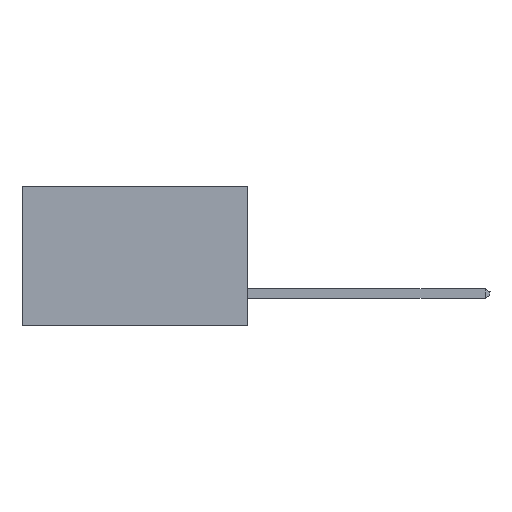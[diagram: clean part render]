
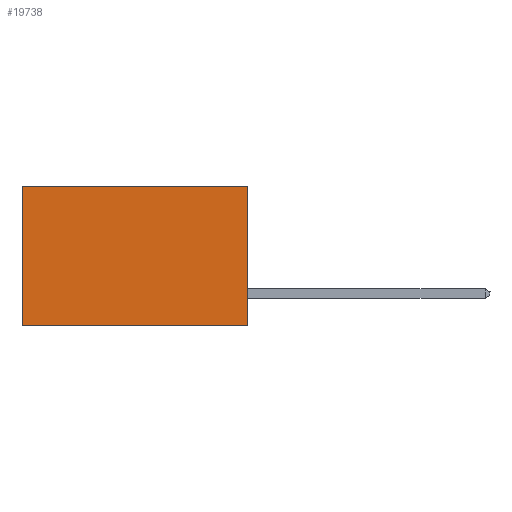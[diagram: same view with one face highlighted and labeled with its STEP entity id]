
A CAD part, left-side view. The second image highlights one B-rep face of the part: STEP entity #19738.
In plain terms, the highlighted planar face has unit normal (-1, 0, 0).
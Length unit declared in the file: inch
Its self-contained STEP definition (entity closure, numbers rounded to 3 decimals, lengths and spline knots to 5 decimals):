
#159 = VERTEX_POINT ( 'NONE', #23981 ) ;
#995 = AXIS2_PLACEMENT_3D ( 'NONE', #24045, #6636, #4983 ) ;
#1008 = ORIENTED_EDGE ( 'NONE', *, *, #24848, .T. ) ;
#1045 = LINE ( 'NONE', #3459, #1400 ) ;
#1400 = VECTOR ( 'NONE', #20501, 39.37008 ) ;
#1782 = CARTESIAN_POINT ( 'NONE',  ( 0.2615, 0.6, 0. ) ) ;
#3459 = CARTESIAN_POINT ( 'NONE',  ( 0.2615, 0., 0. ) ) ;
#3513 = DIRECTION ( 'NONE',  ( 0., 1., 0. ) ) ;
#3581 = LINE ( 'NONE', #15295, #15845 ) ;
#3632 = VECTOR ( 'NONE', #24100, 39.37008 ) ;
#3699 = CARTESIAN_POINT ( 'NONE',  ( 0.2615, 0., 0. ) ) ;
#4983 = DIRECTION ( 'NONE',  ( 0., 0., -1. ) ) ;
#6206 = ORIENTED_EDGE ( 'NONE', *, *, #22979, .F. ) ;
#6636 = DIRECTION ( 'NONE',  ( 1., 0., 0. ) ) ;
#9293 = VERTEX_POINT ( 'NONE', #14397 ) ;
#9300 = ORIENTED_EDGE ( 'NONE', *, *, #20734, .F. ) ;
#10232 = VERTEX_POINT ( 'NONE', #1782 ) ;
#11342 = EDGE_LOOP ( 'NONE', ( #22647, #9300, #6206, #1008 ) ) ;
#12291 = EDGE_CURVE ( 'NONE', #10232, #9293, #23969, .T. ) ;
#13011 = VECTOR ( 'NONE', #3513, 39.37008 ) ;
#14397 = CARTESIAN_POINT ( 'NONE',  ( 0.2615, 0.6, -0.37 ) ) ;
#14917 = DIRECTION ( 'NONE',  ( 0., 0., -1. ) ) ;
#15228 = LINE ( 'NONE', #20674, #13011 ) ;
#15295 = CARTESIAN_POINT ( 'NONE',  ( 0.2615, 0., -0.37 ) ) ;
#15845 = VECTOR ( 'NONE', #14917, 39.37008 ) ;
#19738 = ADVANCED_FACE ( 'NONE', ( #23922 ), #20147, .F. ) ;
#20147 = PLANE ( 'NONE',  #995 ) ;
#20501 = DIRECTION ( 'NONE',  ( 0., 1., 0. ) ) ;
#20563 = CARTESIAN_POINT ( 'NONE',  ( 0.2615, 0.6, -0.37 ) ) ;
#20674 = CARTESIAN_POINT ( 'NONE',  ( 0.2615, 0., -0.37 ) ) ;
#20734 = EDGE_CURVE ( 'NONE', #159, #9293, #15228, .T. ) ;
#22647 = ORIENTED_EDGE ( 'NONE', *, *, #12291, .T. ) ;
#22940 = VERTEX_POINT ( 'NONE', #3699 ) ;
#22979 = EDGE_CURVE ( 'NONE', #22940, #159, #3581, .T. ) ;
#23922 = FACE_OUTER_BOUND ( 'NONE', #11342, .T. ) ;
#23969 = LINE ( 'NONE', #20563, #3632 ) ;
#23981 = CARTESIAN_POINT ( 'NONE',  ( 0.2615, 0., -0.37 ) ) ;
#24045 = CARTESIAN_POINT ( 'NONE',  ( 0.2615, 0., -0.37 ) ) ;
#24100 = DIRECTION ( 'NONE',  ( 0., 0., -1. ) ) ;
#24848 = EDGE_CURVE ( 'NONE', #22940, #10232, #1045, .T. ) ;
